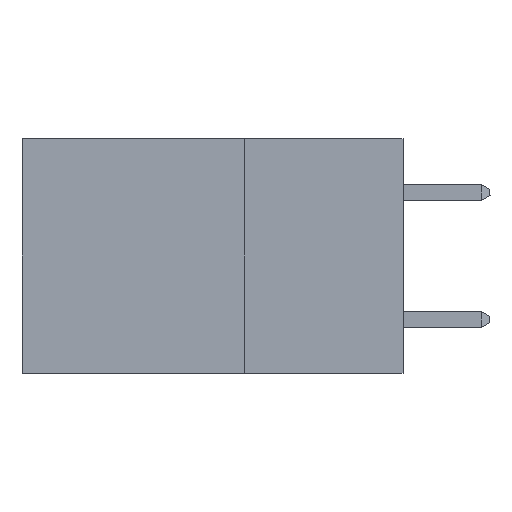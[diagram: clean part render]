
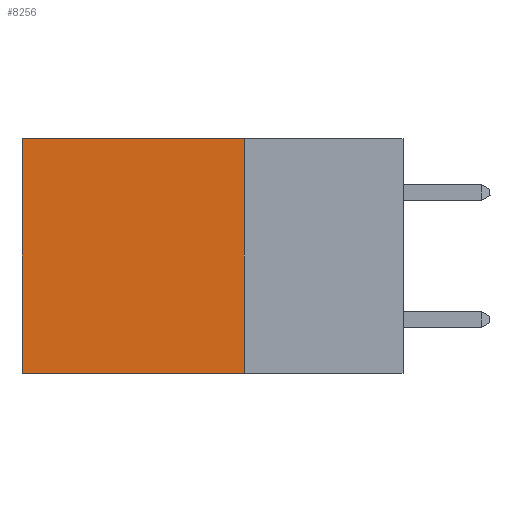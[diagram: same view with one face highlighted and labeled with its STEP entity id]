
A CAD part, left-side view. The second image highlights one B-rep face of the part: STEP entity #8256.
In plain terms, the highlighted planar face has unit normal (-1, 0, 0).
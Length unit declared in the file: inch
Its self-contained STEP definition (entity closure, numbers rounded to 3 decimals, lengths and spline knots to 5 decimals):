
#117 = VERTEX_POINT ( 'NONE', #24930 ) ;
#2509 = DIRECTION ( 'NONE',  ( 0., 0., -1. ) ) ;
#3083 = LINE ( 'NONE', #3289, #29650 ) ;
#3289 = CARTESIAN_POINT ( 'NONE',  ( 0.2875, 0.25, 0. ) ) ;
#6354 = CARTESIAN_POINT ( 'NONE',  ( 0.2875, 0.6, 0. ) ) ;
#8256 = ADVANCED_FACE ( 'NONE', ( #20551 ), #14366, .F. ) ;
#8640 = ORIENTED_EDGE ( 'NONE', *, *, #37887, .F. ) ;
#8703 = ORIENTED_EDGE ( 'NONE', *, *, #15261, .T. ) ;
#9483 = VECTOR ( 'NONE', #2509, 39.37008 ) ;
#9705 = EDGE_LOOP ( 'NONE', ( #28702, #19215, #8640, #8703 ) ) ;
#10602 = VERTEX_POINT ( 'NONE', #12068 ) ;
#12068 = CARTESIAN_POINT ( 'NONE',  ( 0.2875, 0.25, 0. ) ) ;
#13298 = CARTESIAN_POINT ( 'NONE',  ( 0.2875, 0.6, 0. ) ) ;
#14366 = PLANE ( 'NONE',  #37836 ) ;
#15261 = EDGE_CURVE ( 'NONE', #10602, #32099, #3083, .T. ) ;
#16015 = DIRECTION ( 'NONE',  ( 0., 1., 0. ) ) ;
#16603 = VECTOR ( 'NONE', #29834, 39.37008 ) ;
#17264 = DIRECTION ( 'NONE',  ( 0., 0., -1. ) ) ;
#17311 = CARTESIAN_POINT ( 'NONE',  ( 0.2875, 0.25, -0.37 ) ) ;
#19215 = ORIENTED_EDGE ( 'NONE', *, *, #31302, .F. ) ;
#19893 = LINE ( 'NONE', #13298, #22538 ) ;
#20194 = LINE ( 'NONE', #17311, #16603 ) ;
#20551 = FACE_OUTER_BOUND ( 'NONE', #9705, .T. ) ;
#21621 = LINE ( 'NONE', #27168, #9483 ) ;
#22538 = VECTOR ( 'NONE', #25834, 39.37008 ) ;
#24241 = DIRECTION ( 'NONE',  ( 1., 0., 0. ) ) ;
#24930 = CARTESIAN_POINT ( 'NONE',  ( 0.2875, 0.6, -0.37 ) ) ;
#25834 = DIRECTION ( 'NONE',  ( 0., 0., -1. ) ) ;
#27168 = CARTESIAN_POINT ( 'NONE',  ( 0.2875, 0.25, 0. ) ) ;
#28702 = ORIENTED_EDGE ( 'NONE', *, *, #29788, .T. ) ;
#29650 = VECTOR ( 'NONE', #16015, 39.37008 ) ;
#29788 = EDGE_CURVE ( 'NONE', #32099, #117, #19893, .T. ) ;
#29834 = DIRECTION ( 'NONE',  ( 0., 1., 0. ) ) ;
#30603 = CARTESIAN_POINT ( 'NONE',  ( 0.2875, 0.25, 0. ) ) ;
#31302 = EDGE_CURVE ( 'NONE', #39714, #117, #20194, .T. ) ;
#32099 = VERTEX_POINT ( 'NONE', #6354 ) ;
#33665 = CARTESIAN_POINT ( 'NONE',  ( 0.2875, 0.25, -0.37 ) ) ;
#37836 = AXIS2_PLACEMENT_3D ( 'NONE', #30603, #24241, #17264 ) ;
#37887 = EDGE_CURVE ( 'NONE', #10602, #39714, #21621, .T. ) ;
#39714 = VERTEX_POINT ( 'NONE', #33665 ) ;
